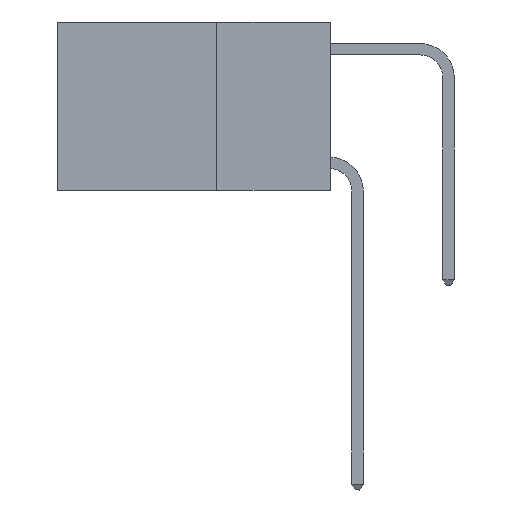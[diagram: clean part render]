
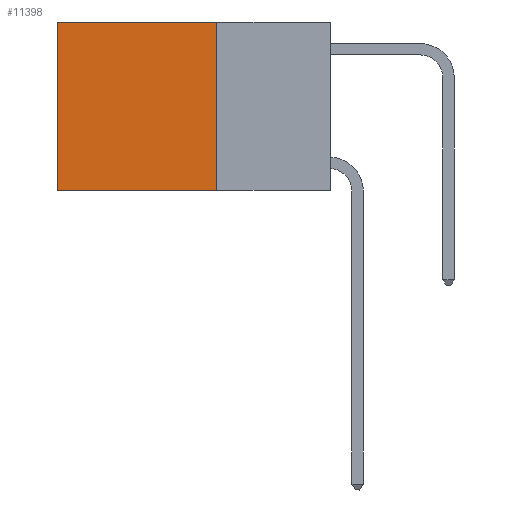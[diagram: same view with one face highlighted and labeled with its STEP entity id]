
A CAD part, left-side view. The second image highlights one B-rep face of the part: STEP entity #11398.
In plain terms, the highlighted planar face has unit normal (-1, 0, 0).
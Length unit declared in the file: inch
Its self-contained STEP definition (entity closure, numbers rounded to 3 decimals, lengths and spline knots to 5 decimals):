
#305 = EDGE_CURVE ( 'NONE', #16881, #5657, #5555, .T. ) ;
#377 = EDGE_CURVE ( 'NONE', #5288, #16881, #17613, .T. ) ;
#809 = VECTOR ( 'NONE', #15651, 39.37008 ) ;
#996 = ORIENTED_EDGE ( 'NONE', *, *, #4241, .F. ) ;
#1228 = VECTOR ( 'NONE', #6823, 39.37008 ) ;
#1537 = CARTESIAN_POINT ( 'NONE',  ( 0.2625, 0.25, 0. ) ) ;
#2337 = LINE ( 'NONE', #16968, #16105 ) ;
#4241 = EDGE_CURVE ( 'NONE', #5288, #5866, #7927, .T. ) ;
#5288 = VERTEX_POINT ( 'NONE', #5582 ) ;
#5408 = CARTESIAN_POINT ( 'NONE',  ( 0.2625, 0.6, 0. ) ) ;
#5555 = LINE ( 'NONE', #5408, #1228 ) ;
#5582 = CARTESIAN_POINT ( 'NONE',  ( 0.2625, 0.25, 0. ) ) ;
#5657 = VERTEX_POINT ( 'NONE', #17611 ) ;
#5866 = VERTEX_POINT ( 'NONE', #15173 ) ;
#6823 = DIRECTION ( 'NONE',  ( 0., 0., -1. ) ) ;
#7847 = DIRECTION ( 'NONE',  ( 0., 0., -1. ) ) ;
#7927 = LINE ( 'NONE', #1537, #9849 ) ;
#8243 = EDGE_CURVE ( 'NONE', #5866, #5657, #2337, .T. ) ;
#8693 = DIRECTION ( 'NONE',  ( 0., 1., 0. ) ) ;
#9849 = VECTOR ( 'NONE', #15128, 39.37008 ) ;
#10177 = AXIS2_PLACEMENT_3D ( 'NONE', #16237, #14952, #7847 ) ;
#11298 = ORIENTED_EDGE ( 'NONE', *, *, #305, .T. ) ;
#11398 = ADVANCED_FACE ( 'NONE', ( #12559 ), #12058, .F. ) ;
#11823 = CARTESIAN_POINT ( 'NONE',  ( 0.2625, 0.6, 0. ) ) ;
#12058 = PLANE ( 'NONE',  #10177 ) ;
#12559 = FACE_OUTER_BOUND ( 'NONE', #17428, .T. ) ;
#13088 = ORIENTED_EDGE ( 'NONE', *, *, #377, .T. ) ;
#14952 = DIRECTION ( 'NONE',  ( 1., 0., 0. ) ) ;
#15128 = DIRECTION ( 'NONE',  ( 0., 0., -1. ) ) ;
#15173 = CARTESIAN_POINT ( 'NONE',  ( 0.2625, 0.25, -0.37 ) ) ;
#15651 = DIRECTION ( 'NONE',  ( 0., 1., 0. ) ) ;
#16105 = VECTOR ( 'NONE', #8693, 39.37008 ) ;
#16237 = CARTESIAN_POINT ( 'NONE',  ( 0.2625, 0.25, 0. ) ) ;
#16433 = ORIENTED_EDGE ( 'NONE', *, *, #8243, .F. ) ;
#16881 = VERTEX_POINT ( 'NONE', #11823 ) ;
#16943 = CARTESIAN_POINT ( 'NONE',  ( 0.2625, 0.25, 0. ) ) ;
#16968 = CARTESIAN_POINT ( 'NONE',  ( 0.2625, 0.25, -0.37 ) ) ;
#17428 = EDGE_LOOP ( 'NONE', ( #11298, #16433, #996, #13088 ) ) ;
#17611 = CARTESIAN_POINT ( 'NONE',  ( 0.2625, 0.6, -0.37 ) ) ;
#17613 = LINE ( 'NONE', #16943, #809 ) ;
